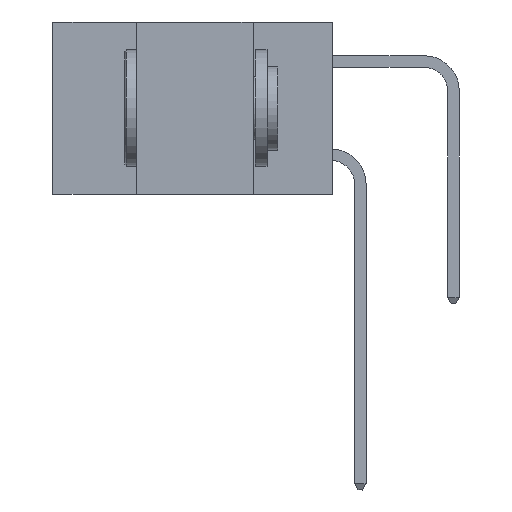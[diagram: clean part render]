
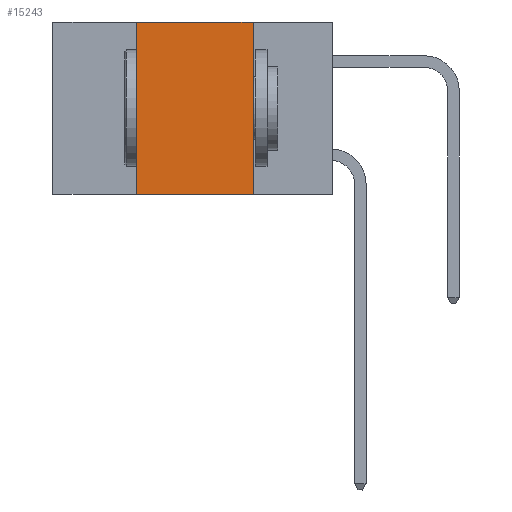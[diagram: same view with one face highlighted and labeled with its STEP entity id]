
A CAD part, left-side view. The second image highlights one B-rep face of the part: STEP entity #15243.
In plain terms, the highlighted planar face has unit normal (-1, 0, 0).
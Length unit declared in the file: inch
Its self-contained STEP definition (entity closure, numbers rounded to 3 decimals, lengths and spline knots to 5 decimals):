
#219 = DIRECTION ( 'NONE',  ( 0., 0., -1. ) ) ;
#332 = DIRECTION ( 'NONE',  ( 0., -1., 0. ) ) ;
#672 = CARTESIAN_POINT ( 'NONE',  ( 0., 0.42, 0. ) ) ;
#694 = CARTESIAN_POINT ( 'NONE',  ( 0., 0.6, 0. ) ) ;
#704 = VECTOR ( 'NONE', #8017, 39.37008 ) ;
#2391 = DIRECTION ( 'NONE',  ( 0., 0., -1. ) ) ;
#2519 = CARTESIAN_POINT ( 'NONE',  ( 0., 0.17, 0. ) ) ;
#2981 = CARTESIAN_POINT ( 'NONE',  ( 0., 0.6, -0.37 ) ) ;
#3091 = LINE ( 'NONE', #14398, #15992 ) ;
#3663 = VERTEX_POINT ( 'NONE', #21496 ) ;
#3668 = ORIENTED_EDGE ( 'NONE', *, *, #11983, .F. ) ;
#3996 = EDGE_LOOP ( 'NONE', ( #18118, #3668, #21006, #19076 ) ) ;
#4261 = LINE ( 'NONE', #8693, #12665 ) ;
#6180 = LINE ( 'NONE', #2981, #704 ) ;
#6839 = VERTEX_POINT ( 'NONE', #2519 ) ;
#7084 = VERTEX_POINT ( 'NONE', #11472 ) ;
#7328 = PLANE ( 'NONE',  #20163 ) ;
#8017 = DIRECTION ( 'NONE',  ( 0., -1., 0. ) ) ;
#8693 = CARTESIAN_POINT ( 'NONE',  ( 0., 0.6, 0. ) ) ;
#9361 = DIRECTION ( 'NONE',  ( 0., 0., 1. ) ) ;
#9489 = EDGE_CURVE ( 'NONE', #3663, #7084, #6180, .T. ) ;
#11472 = CARTESIAN_POINT ( 'NONE',  ( 0., 0.17, -0.37 ) ) ;
#11983 = EDGE_CURVE ( 'NONE', #16190, #6839, #4261, .T. ) ;
#12384 = DIRECTION ( 'NONE',  ( 1., 0., 0. ) ) ;
#12665 = VECTOR ( 'NONE', #332, 39.37008 ) ;
#13367 = FACE_OUTER_BOUND ( 'NONE', #3996, .T. ) ;
#13655 = CARTESIAN_POINT ( 'NONE',  ( 0., 0.17, 0. ) ) ;
#14398 = CARTESIAN_POINT ( 'NONE',  ( 0., 0.42, 0. ) ) ;
#15243 = ADVANCED_FACE ( 'NONE', ( #13367 ), #7328, .F. ) ;
#15992 = VECTOR ( 'NONE', #9361, 39.37008 ) ;
#16190 = VERTEX_POINT ( 'NONE', #672 ) ;
#16311 = EDGE_CURVE ( 'NONE', #3663, #16190, #3091, .T. ) ;
#17662 = VECTOR ( 'NONE', #219, 39.37008 ) ;
#18118 = ORIENTED_EDGE ( 'NONE', *, *, #19578, .F. ) ;
#18156 = LINE ( 'NONE', #13655, #17662 ) ;
#19076 = ORIENTED_EDGE ( 'NONE', *, *, #9489, .T. ) ;
#19578 = EDGE_CURVE ( 'NONE', #6839, #7084, #18156, .T. ) ;
#20163 = AXIS2_PLACEMENT_3D ( 'NONE', #694, #12384, #2391 ) ;
#21006 = ORIENTED_EDGE ( 'NONE', *, *, #16311, .F. ) ;
#21496 = CARTESIAN_POINT ( 'NONE',  ( 0., 0.42, -0.37 ) ) ;
